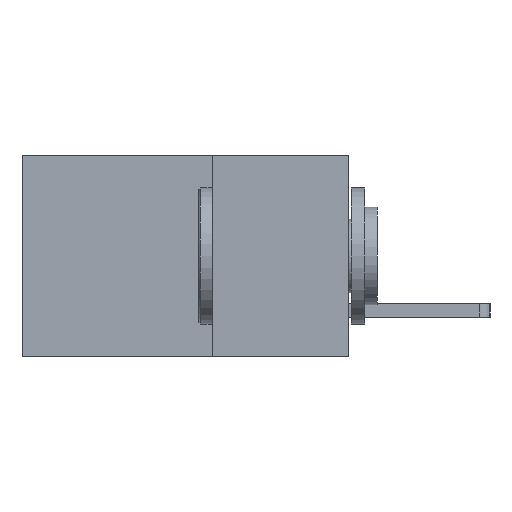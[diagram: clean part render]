
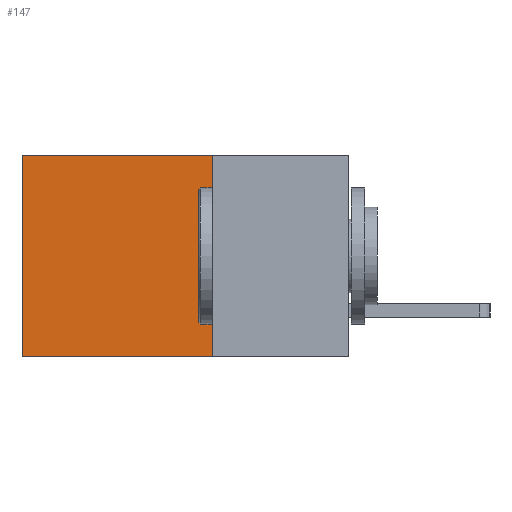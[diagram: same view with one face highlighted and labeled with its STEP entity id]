
A CAD part, left-side view. The second image highlights one B-rep face of the part: STEP entity #147.
In plain terms, the highlighted planar face has unit normal (-1, 0, 0).
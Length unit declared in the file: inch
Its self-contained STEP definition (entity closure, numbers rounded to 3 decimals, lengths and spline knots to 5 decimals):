
#115 = VECTOR ( 'NONE', #7941, 39.37008 ) ;
#118 = LINE ( 'NONE', #7890, #8366 ) ;
#124 = VECTOR ( 'NONE', #5812, 39.37008 ) ;
#147 = ADVANCED_FACE ( 'NONE', ( #4031 ), #8876, .F. ) ;
#595 = DIRECTION ( 'NONE',  ( 0., 0., -1. ) ) ;
#715 = LINE ( 'NONE', #8901, #8961 ) ;
#1234 = EDGE_CURVE ( 'NONE', #6313, #6386, #118, .T. ) ;
#1675 = DIRECTION ( 'NONE',  ( 0., 0., -1. ) ) ;
#2001 = ORIENTED_EDGE ( 'NONE', *, *, #9272, .F. ) ;
#2271 = EDGE_CURVE ( 'NONE', #6416, #6313, #715, .T. ) ;
#2569 = CARTESIAN_POINT ( 'NONE',  ( 0.298, 0.25, -0.37 ) ) ;
#2631 = DIRECTION ( 'NONE',  ( 1., 0., 0. ) ) ;
#3115 = ORIENTED_EDGE ( 'NONE', *, *, #8847, .F. ) ;
#3116 = CARTESIAN_POINT ( 'NONE',  ( 0.298, 0.25, 0. ) ) ;
#3255 = CARTESIAN_POINT ( 'NONE',  ( 0.298, 0.25, 0. ) ) ;
#3965 = CARTESIAN_POINT ( 'NONE',  ( 0.298, 0.6, 0. ) ) ;
#4007 = CARTESIAN_POINT ( 'NONE',  ( 0.298, 0.25, -0.37 ) ) ;
#4031 = FACE_OUTER_BOUND ( 'NONE', #5884, .T. ) ;
#4864 = CARTESIAN_POINT ( 'NONE',  ( 0.298, 0.25, 0. ) ) ;
#4904 = ORIENTED_EDGE ( 'NONE', *, *, #2271, .T. ) ;
#5662 = CARTESIAN_POINT ( 'NONE',  ( 0.298, 0.6, -0.37 ) ) ;
#5812 = DIRECTION ( 'NONE',  ( 0., 1., 0. ) ) ;
#5884 = EDGE_LOOP ( 'NONE', ( #7634, #3115, #2001, #4904 ) ) ;
#6313 = VERTEX_POINT ( 'NONE', #3965 ) ;
#6386 = VERTEX_POINT ( 'NONE', #5662 ) ;
#6416 = VERTEX_POINT ( 'NONE', #3255 ) ;
#7634 = ORIENTED_EDGE ( 'NONE', *, *, #1234, .T. ) ;
#7736 = AXIS2_PLACEMENT_3D ( 'NONE', #4864, #2631, #595 ) ;
#7890 = CARTESIAN_POINT ( 'NONE',  ( 0.298, 0.6, 0. ) ) ;
#7941 = DIRECTION ( 'NONE',  ( 0., 0., -1. ) ) ;
#8363 = LINE ( 'NONE', #3116, #115 ) ;
#8366 = VECTOR ( 'NONE', #1675, 39.37008 ) ;
#8373 = LINE ( 'NONE', #2569, #124 ) ;
#8626 = DIRECTION ( 'NONE',  ( 0., 1., 0. ) ) ;
#8813 = VERTEX_POINT ( 'NONE', #4007 ) ;
#8847 = EDGE_CURVE ( 'NONE', #8813, #6386, #8373, .T. ) ;
#8876 = PLANE ( 'NONE',  #7736 ) ;
#8901 = CARTESIAN_POINT ( 'NONE',  ( 0.298, 0.25, 0. ) ) ;
#8961 = VECTOR ( 'NONE', #8626, 39.37008 ) ;
#9272 = EDGE_CURVE ( 'NONE', #6416, #8813, #8363, .T. ) ;
